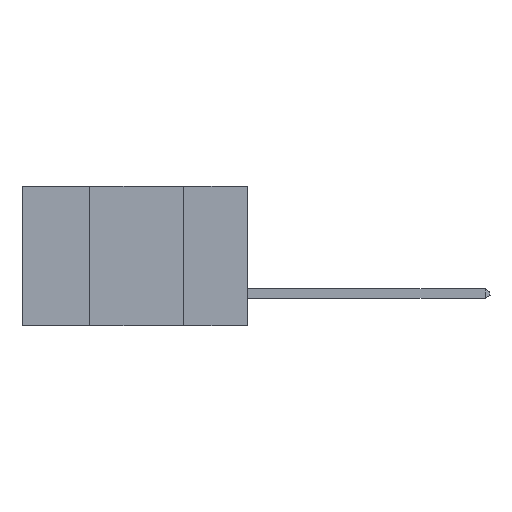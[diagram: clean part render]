
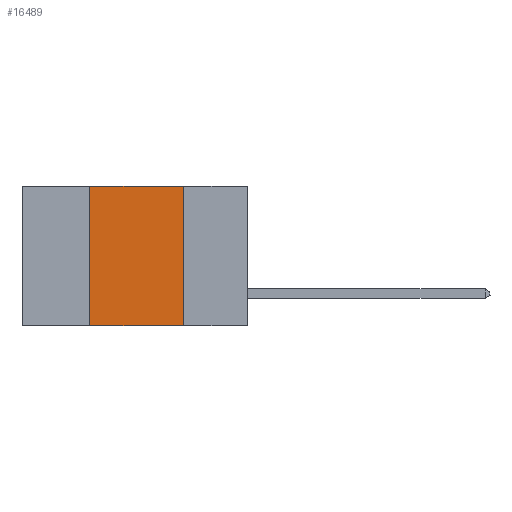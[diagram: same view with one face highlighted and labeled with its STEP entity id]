
A CAD part, left-side view. The second image highlights one B-rep face of the part: STEP entity #16489.
In plain terms, the highlighted planar face has unit normal (-1, 0, 0).
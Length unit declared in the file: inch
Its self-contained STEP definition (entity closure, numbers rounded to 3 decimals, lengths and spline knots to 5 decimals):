
#57 = VERTEX_POINT ( 'NONE', #6435 ) ;
#461 = LINE ( 'NONE', #912, #5845 ) ;
#912 = CARTESIAN_POINT ( 'NONE',  ( 0., 0.17, 0. ) ) ;
#1014 = DIRECTION ( 'NONE',  ( 1., 0., 0. ) ) ;
#2249 = LINE ( 'NONE', #22274, #8934 ) ;
#2577 = EDGE_CURVE ( 'NONE', #10367, #17355, #461, .T. ) ;
#3045 = EDGE_CURVE ( 'NONE', #57, #10367, #23996, .T. ) ;
#3165 = DIRECTION ( 'NONE',  ( 0., -1., 0. ) ) ;
#3724 = ORIENTED_EDGE ( 'NONE', *, *, #2577, .F. ) ;
#4998 = FACE_OUTER_BOUND ( 'NONE', #12111, .T. ) ;
#5845 = VECTOR ( 'NONE', #15858, 39.37008 ) ;
#6435 = CARTESIAN_POINT ( 'NONE',  ( 0., 0.42, 0. ) ) ;
#7871 = ORIENTED_EDGE ( 'NONE', *, *, #23314, .F. ) ;
#8134 = DIRECTION ( 'NONE',  ( 0., -1., 0. ) ) ;
#8934 = VECTOR ( 'NONE', #3165, 39.37008 ) ;
#10367 = VERTEX_POINT ( 'NONE', #17924 ) ;
#11040 = CARTESIAN_POINT ( 'NONE',  ( 0., 0.42, 0. ) ) ;
#12111 = EDGE_LOOP ( 'NONE', ( #3724, #27417, #7871, #22032 ) ) ;
#12224 = CARTESIAN_POINT ( 'NONE',  ( 0., 0.42, -0.37 ) ) ;
#12266 = LINE ( 'NONE', #11040, #26264 ) ;
#15858 = DIRECTION ( 'NONE',  ( 0., 0., -1. ) ) ;
#16034 = PLANE ( 'NONE',  #20194 ) ;
#16489 = ADVANCED_FACE ( 'NONE', ( #4998 ), #16034, .F. ) ;
#17355 = VERTEX_POINT ( 'NONE', #23774 ) ;
#17924 = CARTESIAN_POINT ( 'NONE',  ( 0., 0.17, 0. ) ) ;
#18072 = DIRECTION ( 'NONE',  ( 0., 0., -1. ) ) ;
#18709 = VECTOR ( 'NONE', #8134, 39.37008 ) ;
#20194 = AXIS2_PLACEMENT_3D ( 'NONE', #20395, #1014, #18072 ) ;
#20395 = CARTESIAN_POINT ( 'NONE',  ( 0., 0.6, 0. ) ) ;
#22032 = ORIENTED_EDGE ( 'NONE', *, *, #22954, .T. ) ;
#22274 = CARTESIAN_POINT ( 'NONE',  ( 0., 0.6, -0.37 ) ) ;
#22954 = EDGE_CURVE ( 'NONE', #24690, #17355, #2249, .T. ) ;
#23314 = EDGE_CURVE ( 'NONE', #24690, #57, #12266, .T. ) ;
#23774 = CARTESIAN_POINT ( 'NONE',  ( 0., 0.17, -0.37 ) ) ;
#23996 = LINE ( 'NONE', #25184, #18709 ) ;
#24690 = VERTEX_POINT ( 'NONE', #12224 ) ;
#25184 = CARTESIAN_POINT ( 'NONE',  ( 0., 0.6, 0. ) ) ;
#25969 = DIRECTION ( 'NONE',  ( 0., 0., 1. ) ) ;
#26264 = VECTOR ( 'NONE', #25969, 39.37008 ) ;
#27417 = ORIENTED_EDGE ( 'NONE', *, *, #3045, .F. ) ;
